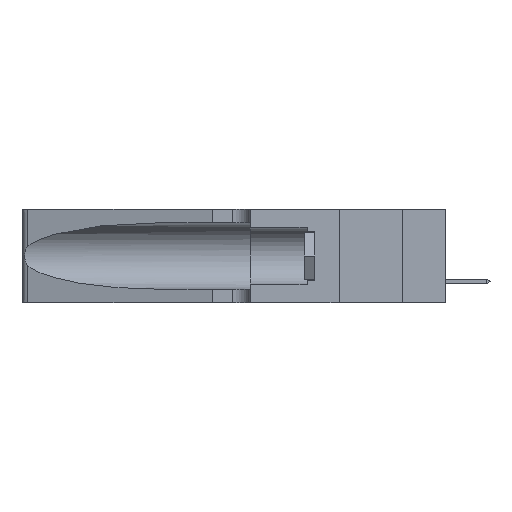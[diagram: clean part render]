
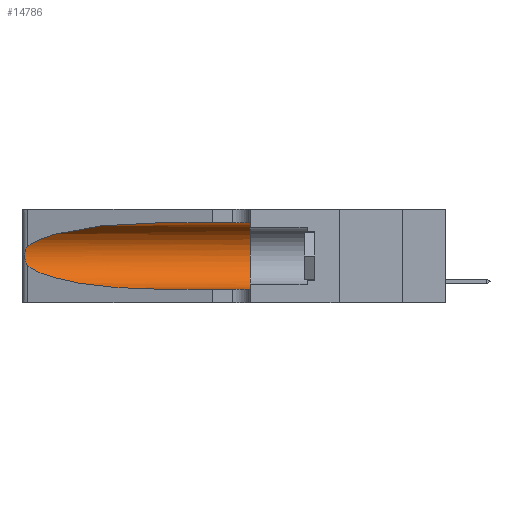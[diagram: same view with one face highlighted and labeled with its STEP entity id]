
A CAD part, left-side view. The second image highlights one B-rep face of the part: STEP entity #14786.
In plain terms, the highlighted cylindrical face has radius 3.308 mm (diameter 6.617 mm), a partial arc.
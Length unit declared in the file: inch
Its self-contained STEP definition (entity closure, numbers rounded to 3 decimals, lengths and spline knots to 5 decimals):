
#246 = DIRECTION ( 'NONE',  ( 0., 0., 1. ) ) ;
#361 = CARTESIAN_POINT ( 'NONE',  ( 0.25854, 1.2359, 0.20912 ) ) ;
#368 = EDGE_LOOP ( 'NONE', ( #15316, #26055, #11740, #12460, #21234, #3639 ) ) ;
#606 = CARTESIAN_POINT ( 'NONE',  ( 0.25555, 1.22993, 0.14849 ) ) ;
#2231 = CARTESIAN_POINT ( 'NONE',  ( 0.25487, 1.22718, 0.14631 ) ) ;
#2748 = CARTESIAN_POINT ( 'NONE',  ( 0.26018, 1.23835, 0.19895 ) ) ;
#3299 = CARTESIAN_POINT ( 'NONE',  ( 0.2373, 1.15595, 0.08982 ) ) ;
#3556 = CARTESIAN_POINT ( 'NONE',  ( 0.1305, 1.61858, 0.05475 ) ) ;
#3639 = ORIENTED_EDGE ( 'NONE', *, *, #15915, .F. ) ;
#3817 = VERTEX_POINT ( 'NONE', #28576 ) ;
#4004 = VERTEX_POINT ( 'NONE', #29311 ) ;
#6051 = CARTESIAN_POINT ( 'NONE',  ( 0.25787, 1.23484, 0.2124 ) ) ;
#6137 = CARTESIAN_POINT ( 'NONE',  ( 0.1305, 0.72297, 0.05475 ) ) ;
#8937 = B_SPLINE_CURVE_WITH_KNOTS ( 'NONE', 3,
 ( #19688, #36023, #22769, #6051, #361, #2748, #14312, #28542, #12336, #29040, #17538, #23133, #606, #28914 ),
 .UNSPECIFIED., .F., .F.,
 ( 4, 2, 2, 2, 2, 2, 4 ),
 ( 0., 0.00027, 0.00053, 0.00107, 0.0016, 0.00187, 0.00214 ),
 .UNSPECIFIED. ) ;
#10220 = CARTESIAN_POINT ( 'NONE',  ( 0.1305, 0.72297, 0.31525 ) ) ;
#11703 = EDGE_CURVE ( 'NONE', #18483, #3817, #34015, .T. ) ;
#11740 = ORIENTED_EDGE ( 'NONE', *, *, #17089, .T. ) ;
#12336 = CARTESIAN_POINT ( 'NONE',  ( 0.26017, 1.23833, 0.17102 ) ) ;
#12460 = ORIENTED_EDGE ( 'NONE', *, *, #35706, .T. ) ;
#13213 = DIRECTION ( 'NONE',  ( 0., 0., -1. ) ) ;
#13280 = VECTOR ( 'NONE', #26180, 39.37008 ) ;
#13629 = VECTOR ( 'NONE', #22569, 39.37008 ) ;
#14312 = CARTESIAN_POINT ( 'NONE',  ( 0.26075, 1.23896, 0.19203 ) ) ;
#14322 = CARTESIAN_POINT ( 'NONE',  ( 0.1305, 0.35, 0.185 ) ) ;
#14786 = ADVANCED_FACE ( 'NONE', ( #23905 ), #20314, .F. ) ;
#15316 = ORIENTED_EDGE ( 'NONE', *, *, #11703, .T. ) ;
#15424 = CARTESIAN_POINT ( 'NONE',  ( 0.1305, 0.72297, 0.31525 ) ) ;
#15915 = EDGE_CURVE ( 'NONE', #18483, #29053, #31682, .T. ) ;
#16748 = CARTESIAN_POINT ( 'NONE',  ( 0.1305, 1.61858, 0.31525 ) ) ;
#17089 = EDGE_CURVE ( 'NONE', #19785, #4004, #34468, .T. ) ;
#17538 = CARTESIAN_POINT ( 'NONE',  ( 0.25789, 1.23486, 0.15765 ) ) ;
#18483 = VERTEX_POINT ( 'NONE', #10220 ) ;
#18704 = CARTESIAN_POINT ( 'NONE',  ( 0.1305, 1.61858, 0.185 ) ) ;
#19688 = CARTESIAN_POINT ( 'NONE',  ( 0.25487, 1.22718, 0.22369 ) ) ;
#19785 = VERTEX_POINT ( 'NONE', #2231 ) ;
#20314 = CYLINDRICAL_SURFACE ( 'NONE', #24841, 0.13025 ) ;
#20878 = CIRCLE ( 'NONE', #28069, 0.13025 ) ;
#21234 = ORIENTED_EDGE ( 'NONE', *, *, #27597, .F. ) ;
#22569 = DIRECTION ( 'NONE',  ( 0., -1., 0. ) ) ;
#22769 = CARTESIAN_POINT ( 'NONE',  ( 0.25639, 1.23184, 0.21858 ) ) ;
#22987 = VERTEX_POINT ( 'NONE', #35567 ) ;
#23091 = CARTESIAN_POINT ( 'NONE',  ( 0.18966, 0.96281, 0.05475 ) ) ;
#23133 = CARTESIAN_POINT ( 'NONE',  ( 0.25639, 1.23186, 0.15144 ) ) ;
#23905 = FACE_OUTER_BOUND ( 'NONE', #368, .T. ) ;
#24841 = AXIS2_PLACEMENT_3D ( 'NONE', #18704, #30162, #13213 ) ;
#25700 = LINE ( 'NONE', #3556, #13280 ) ;
#26055 = ORIENTED_EDGE ( 'NONE', *, *, #29995, .T. ) ;
#26180 = DIRECTION ( 'NONE',  ( 0., -1., 0. ) ) ;
#27597 = EDGE_CURVE ( 'NONE', #29053, #22987, #20878, .T. ) ;
#28069 = AXIS2_PLACEMENT_3D ( 'NONE', #14322, #34047, #246 ) ;
#28542 = CARTESIAN_POINT ( 'NONE',  ( 0.26075, 1.23896, 0.178 ) ) ;
#28576 = CARTESIAN_POINT ( 'NONE',  ( 0.25487, 1.22718, 0.22369 ) ) ;
#28914 = CARTESIAN_POINT ( 'NONE',  ( 0.25487, 1.22718, 0.14631 ) ) ;
#29003 = CARTESIAN_POINT ( 'NONE',  ( 0.25487, 1.22718, 0.14631 ) ) ;
#29040 = CARTESIAN_POINT ( 'NONE',  ( 0.25856, 1.23593, 0.16098 ) ) ;
#29053 = VERTEX_POINT ( 'NONE', #34097 ) ;
#29311 = CARTESIAN_POINT ( 'NONE',  ( 0.1305, 0.72297, 0.05475 ) ) ;
#29408 = CARTESIAN_POINT ( 'NONE',  ( 0.18966, 0.96281, 0.31525 ) ) ;
#29995 = EDGE_CURVE ( 'NONE', #3817, #19785, #8937, .T. ) ;
#30162 = DIRECTION ( 'NONE',  ( 0., -1., 0. ) ) ;
#31682 = LINE ( 'NONE', #16748, #13629 ) ;
#34015 =( BOUNDED_CURVE ( )  B_SPLINE_CURVE ( 3, ( #15424, #29408, #34772, #35021 ),
 .UNSPECIFIED., .F., .F. ) 
 B_SPLINE_CURVE_WITH_KNOTS ( ( 4, 4 ),
 ( 1.5708, 2.84003 ),
 .UNSPECIFIED. ) 
 CURVE ( )  GEOMETRIC_REPRESENTATION_ITEM ( )  RATIONAL_B_SPLINE_CURVE ( ( 1., 0.87, 0.87, 1. ) ) 
 REPRESENTATION_ITEM ( '' )  );
#34047 = DIRECTION ( 'NONE',  ( 0., 1., 0. ) ) ;
#34097 = CARTESIAN_POINT ( 'NONE',  ( 0.1305, 0.35, 0.31525 ) ) ;
#34468 =( BOUNDED_CURVE ( )  B_SPLINE_CURVE ( 3, ( #29003, #3299, #23091, #6137 ),
 .UNSPECIFIED., .F., .F. ) 
 B_SPLINE_CURVE_WITH_KNOTS ( ( 4, 4 ),
 ( 3.44316, 4.71239 ),
 .UNSPECIFIED. ) 
 CURVE ( )  GEOMETRIC_REPRESENTATION_ITEM ( )  RATIONAL_B_SPLINE_CURVE ( ( 1., 0.87, 0.87, 1. ) ) 
 REPRESENTATION_ITEM ( '' )  );
#34772 = CARTESIAN_POINT ( 'NONE',  ( 0.2373, 1.15595, 0.28018 ) ) ;
#35021 = CARTESIAN_POINT ( 'NONE',  ( 0.25487, 1.22718, 0.22369 ) ) ;
#35567 = CARTESIAN_POINT ( 'NONE',  ( 0.1305, 0.35, 0.05475 ) ) ;
#35706 = EDGE_CURVE ( 'NONE', #4004, #22987, #25700, .T. ) ;
#36023 = CARTESIAN_POINT ( 'NONE',  ( 0.25555, 1.22994, 0.2215 ) ) ;
